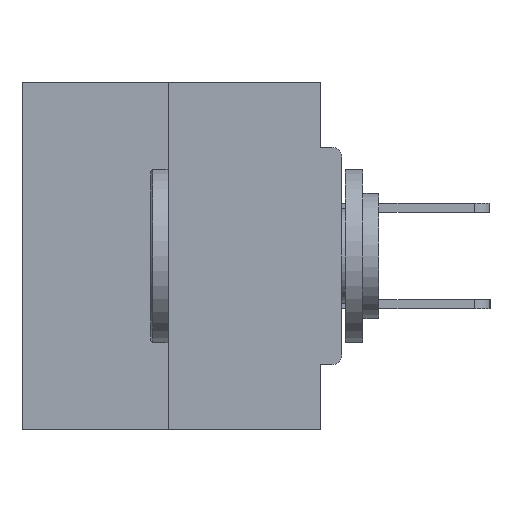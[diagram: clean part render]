
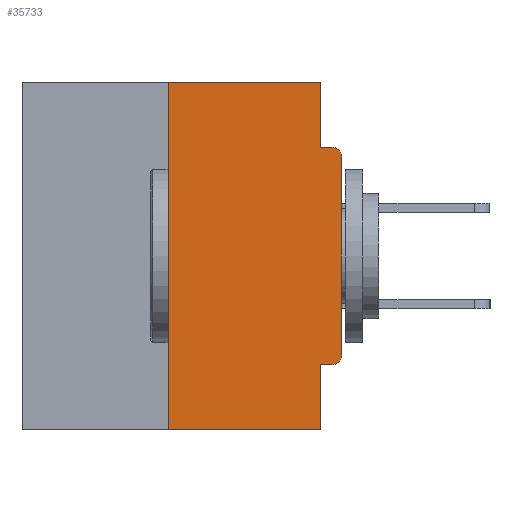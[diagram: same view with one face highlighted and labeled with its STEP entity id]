
A CAD part, left-side view. The second image highlights one B-rep face of the part: STEP entity #35733.
In plain terms, the highlighted planar face has unit normal (-1, 0, 0).
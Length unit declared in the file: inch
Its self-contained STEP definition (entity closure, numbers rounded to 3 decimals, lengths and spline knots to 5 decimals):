
#366 = CARTESIAN_POINT ( 'NONE',  ( 0., 0.25, -0.5 ) ) ;
#874 = FACE_OUTER_BOUND ( 'NONE', #8593, .T. ) ;
#918 = EDGE_CURVE ( 'NONE', #27079, #1662, #25189, .T. ) ;
#964 = LINE ( 'NONE', #3805, #31888 ) ;
#1297 = CARTESIAN_POINT ( 'NONE',  ( 0., 0.46, 0. ) ) ;
#1327 = CARTESIAN_POINT ( 'NONE',  ( 0., 0.46, 0. ) ) ;
#1456 = CARTESIAN_POINT ( 'NONE',  ( 0., 0., -0.0935 ) ) ;
#1655 = VECTOR ( 'NONE', #14501, 39.37008 ) ;
#1662 = VERTEX_POINT ( 'NONE', #1995 ) ;
#1881 = LINE ( 'NONE', #1297, #15983 ) ;
#1995 = CARTESIAN_POINT ( 'NONE',  ( 0., 0.031, -0.4065 ) ) ;
#2052 = VERTEX_POINT ( 'NONE', #3942 ) ;
#2305 = ORIENTED_EDGE ( 'NONE', *, *, #918, .F. ) ;
#2722 = CARTESIAN_POINT ( 'NONE',  ( 0., 0.015, -0.1085 ) ) ;
#2799 = DIRECTION ( 'NONE',  ( 0., 0., -1. ) ) ;
#3365 = VERTEX_POINT ( 'NONE', #32099 ) ;
#3657 = DIRECTION ( 'NONE',  ( 0., 0., -1. ) ) ;
#3805 = CARTESIAN_POINT ( 'NONE',  ( 0., 0., 0. ) ) ;
#3942 = CARTESIAN_POINT ( 'NONE',  ( 0., 0.031, -0.0935 ) ) ;
#4618 = VECTOR ( 'NONE', #7460, 39.37008 ) ;
#5414 = LINE ( 'NONE', #14110, #1655 ) ;
#5469 = DIRECTION ( 'NONE',  ( 0., 0., -1. ) ) ;
#5764 = CARTESIAN_POINT ( 'NONE',  ( 0., 0.031, -0.5 ) ) ;
#6102 = ORIENTED_EDGE ( 'NONE', *, *, #16296, .F. ) ;
#7352 = VECTOR ( 'NONE', #38182, 39.37008 ) ;
#7460 = DIRECTION ( 'NONE',  ( 0., -1., 0. ) ) ;
#7799 = CARTESIAN_POINT ( 'NONE',  ( 0., 0.25, 0. ) ) ;
#8454 = CARTESIAN_POINT ( 'NONE',  ( 0., 0.015, -0.3915 ) ) ;
#8593 = EDGE_LOOP ( 'NONE', ( #6102, #14625, #13070, #32620, #2305, #26311, #22883, #35735, #19686, #26399 ) ) ;
#10500 = DIRECTION ( 'NONE',  ( 0., 0., -1. ) ) ;
#10608 = EDGE_CURVE ( 'NONE', #1662, #36052, #32310, .T. ) ;
#11583 = EDGE_CURVE ( 'NONE', #17068, #21852, #30851, .T. ) ;
#12678 = VECTOR ( 'NONE', #2799, 39.37008 ) ;
#13070 = ORIENTED_EDGE ( 'NONE', *, *, #31993, .T. ) ;
#13508 = DIRECTION ( 'NONE',  ( 0., 0., 1. ) ) ;
#14110 = CARTESIAN_POINT ( 'NONE',  ( 0., 0.46, -0.5 ) ) ;
#14501 = DIRECTION ( 'NONE',  ( 0., -1., 0. ) ) ;
#14547 = DIRECTION ( 'NONE',  ( -1., 0., 0. ) ) ;
#14625 = ORIENTED_EDGE ( 'NONE', *, *, #11583, .F. ) ;
#15983 = VECTOR ( 'NONE', #37037, 39.37008 ) ;
#16159 = PLANE ( 'NONE',  #20884 ) ;
#16253 = EDGE_CURVE ( 'NONE', #17168, #29796, #964, .T. ) ;
#16296 = EDGE_CURVE ( 'NONE', #21852, #3365, #1881, .T. ) ;
#17068 = VERTEX_POINT ( 'NONE', #366 ) ;
#17168 = VERTEX_POINT ( 'NONE', #22208 ) ;
#17413 = EDGE_CURVE ( 'NONE', #29796, #32068, #33185, .T. ) ;
#18969 = CARTESIAN_POINT ( 'NONE',  ( 0., 0.015, -0.4065 ) ) ;
#19534 = AXIS2_PLACEMENT_3D ( 'NONE', #2722, #14547, #3657 ) ;
#19686 = ORIENTED_EDGE ( 'NONE', *, *, #27622, .F. ) ;
#19966 = EDGE_CURVE ( 'NONE', #3365, #2052, #35528, .T. ) ;
#20079 = CARTESIAN_POINT ( 'NONE',  ( 0., 0., -0.1085 ) ) ;
#20593 = LINE ( 'NONE', #1456, #4618 ) ;
#20884 = AXIS2_PLACEMENT_3D ( 'NONE', #1327, #31583, #10500 ) ;
#21191 = EDGE_CURVE ( 'NONE', #27079, #17168, #36780, .T. ) ;
#21852 = VERTEX_POINT ( 'NONE', #26790 ) ;
#22208 = CARTESIAN_POINT ( 'NONE',  ( 0., 0., -0.3915 ) ) ;
#22883 = ORIENTED_EDGE ( 'NONE', *, *, #16253, .T. ) ;
#23050 = CARTESIAN_POINT ( 'NONE',  ( 0., 0.031, 0. ) ) ;
#23764 = CARTESIAN_POINT ( 'NONE',  ( 0., 0.031, -0.5 ) ) ;
#25189 = LINE ( 'NONE', #31800, #7352 ) ;
#26311 = ORIENTED_EDGE ( 'NONE', *, *, #21191, .T. ) ;
#26399 = ORIENTED_EDGE ( 'NONE', *, *, #19966, .F. ) ;
#26659 = VECTOR ( 'NONE', #31827, 39.37008 ) ;
#26790 = CARTESIAN_POINT ( 'NONE',  ( 0., 0.25, 0. ) ) ;
#27079 = VERTEX_POINT ( 'NONE', #18969 ) ;
#27622 = EDGE_CURVE ( 'NONE', #2052, #32068, #20593, .T. ) ;
#28546 = DIRECTION ( 'NONE',  ( 0., 0., 1. ) ) ;
#29041 = CARTESIAN_POINT ( 'NONE',  ( 0., 0.015, -0.0935 ) ) ;
#29796 = VERTEX_POINT ( 'NONE', #20079 ) ;
#29939 = VECTOR ( 'NONE', #28546, 39.37008 ) ;
#30851 = LINE ( 'NONE', #7799, #29939 ) ;
#31583 = DIRECTION ( 'NONE',  ( 1., 0., 0. ) ) ;
#31800 = CARTESIAN_POINT ( 'NONE',  ( 0., 0., -0.4065 ) ) ;
#31827 = DIRECTION ( 'NONE',  ( 0., 0., -1. ) ) ;
#31888 = VECTOR ( 'NONE', #13508, 39.37008 ) ;
#31993 = EDGE_CURVE ( 'NONE', #17068, #36052, #5414, .T. ) ;
#32068 = VERTEX_POINT ( 'NONE', #29041 ) ;
#32099 = CARTESIAN_POINT ( 'NONE',  ( 0., 0.031, 0. ) ) ;
#32310 = LINE ( 'NONE', #23764, #12678 ) ;
#32620 = ORIENTED_EDGE ( 'NONE', *, *, #10608, .F. ) ;
#33185 = CIRCLE ( 'NONE', #19534, 0.015 ) ;
#33891 = AXIS2_PLACEMENT_3D ( 'NONE', #8454, #38553, #5469 ) ;
#35528 = LINE ( 'NONE', #23050, #26659 ) ;
#35733 = ADVANCED_FACE ( 'NONE', ( #874 ), #16159, .F. ) ;
#35735 = ORIENTED_EDGE ( 'NONE', *, *, #17413, .T. ) ;
#36052 = VERTEX_POINT ( 'NONE', #5764 ) ;
#36780 = CIRCLE ( 'NONE', #33891, 0.015 ) ;
#37037 = DIRECTION ( 'NONE',  ( 0., -1., 0. ) ) ;
#38182 = DIRECTION ( 'NONE',  ( 0., 1., 0. ) ) ;
#38553 = DIRECTION ( 'NONE',  ( -1., 0., 0. ) ) ;
